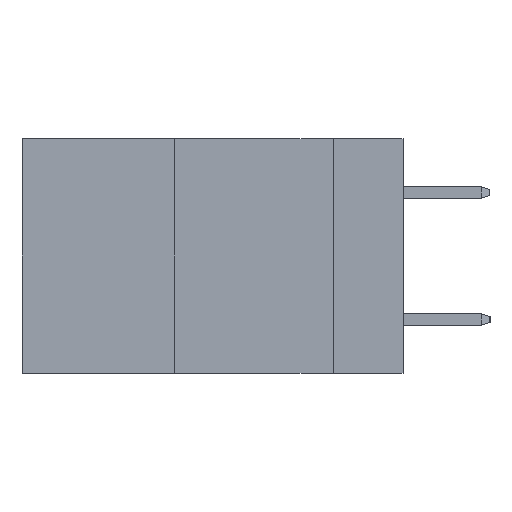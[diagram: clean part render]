
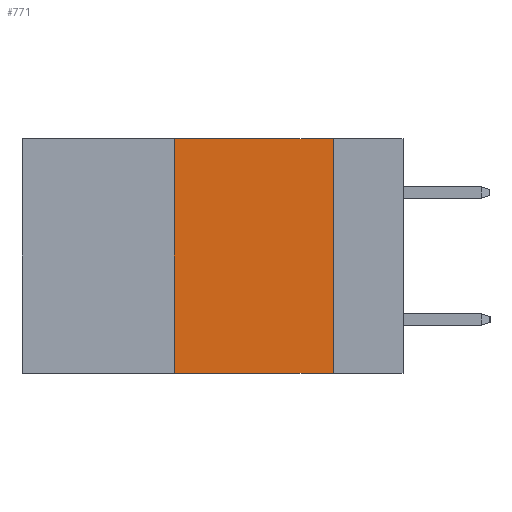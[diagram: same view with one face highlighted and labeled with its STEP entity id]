
A CAD part, left-side view. The second image highlights one B-rep face of the part: STEP entity #771.
In plain terms, the highlighted planar face has unit normal (-1, 0, 0).
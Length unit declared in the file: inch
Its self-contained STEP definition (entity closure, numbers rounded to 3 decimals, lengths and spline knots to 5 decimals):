
#499 = VECTOR ( 'NONE', #4018, 39.37008 ) ;
#771 = ADVANCED_FACE ( 'NONE', ( #8908 ), #3837, .F. ) ;
#1419 = CARTESIAN_POINT ( 'NONE',  ( 0., 0.6, -0.37 ) ) ;
#1892 = AXIS2_PLACEMENT_3D ( 'NONE', #5465, #2021, #5410 ) ;
#1943 = VERTEX_POINT ( 'NONE', #9695 ) ;
#2021 = DIRECTION ( 'NONE',  ( 1., 0., 0. ) ) ;
#2035 = LINE ( 'NONE', #5423, #499 ) ;
#2253 = VECTOR ( 'NONE', #3057, 39.37008 ) ;
#2779 = EDGE_CURVE ( 'NONE', #5441, #8520, #2035, .T. ) ;
#2947 = EDGE_CURVE ( 'NONE', #1943, #5441, #9764, .T. ) ;
#3057 = DIRECTION ( 'NONE',  ( 0., 0., 1. ) ) ;
#3349 = VERTEX_POINT ( 'NONE', #7712 ) ;
#3350 = CARTESIAN_POINT ( 'NONE',  ( 0., 0.11, 0. ) ) ;
#3412 = CARTESIAN_POINT ( 'NONE',  ( 0., 0.36, 0. ) ) ;
#3837 = PLANE ( 'NONE',  #1892 ) ;
#3838 = ORIENTED_EDGE ( 'NONE', *, *, #2947, .F. ) ;
#3942 = DIRECTION ( 'NONE',  ( 0., -1., 0. ) ) ;
#4018 = DIRECTION ( 'NONE',  ( 0., -1., 0. ) ) ;
#4461 = CARTESIAN_POINT ( 'NONE',  ( 0., 0.11, 0. ) ) ;
#4588 = EDGE_LOOP ( 'NONE', ( #7533, #6414, #3838, #6266 ) ) ;
#5303 = DIRECTION ( 'NONE',  ( 0., 0., -1. ) ) ;
#5410 = DIRECTION ( 'NONE',  ( 0., 0., -1. ) ) ;
#5423 = CARTESIAN_POINT ( 'NONE',  ( 0., 0.6, 0. ) ) ;
#5441 = VERTEX_POINT ( 'NONE', #3412 ) ;
#5465 = CARTESIAN_POINT ( 'NONE',  ( 0., 0.6, 0. ) ) ;
#5568 = CARTESIAN_POINT ( 'NONE',  ( 0., 0.36, 0. ) ) ;
#6266 = ORIENTED_EDGE ( 'NONE', *, *, #8803, .T. ) ;
#6384 = EDGE_CURVE ( 'NONE', #8520, #3349, #7696, .T. ) ;
#6414 = ORIENTED_EDGE ( 'NONE', *, *, #2779, .F. ) ;
#6454 = VECTOR ( 'NONE', #3942, 39.37008 ) ;
#6580 = LINE ( 'NONE', #1419, #6454 ) ;
#7533 = ORIENTED_EDGE ( 'NONE', *, *, #6384, .F. ) ;
#7696 = LINE ( 'NONE', #4461, #10271 ) ;
#7712 = CARTESIAN_POINT ( 'NONE',  ( 0., 0.11, -0.37 ) ) ;
#8520 = VERTEX_POINT ( 'NONE', #3350 ) ;
#8803 = EDGE_CURVE ( 'NONE', #1943, #3349, #6580, .T. ) ;
#8908 = FACE_OUTER_BOUND ( 'NONE', #4588, .T. ) ;
#9695 = CARTESIAN_POINT ( 'NONE',  ( 0., 0.36, -0.37 ) ) ;
#9764 = LINE ( 'NONE', #5568, #2253 ) ;
#10271 = VECTOR ( 'NONE', #5303, 39.37008 ) ;
